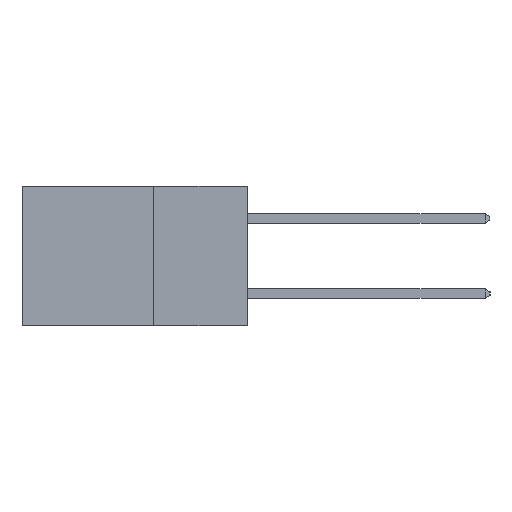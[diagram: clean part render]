
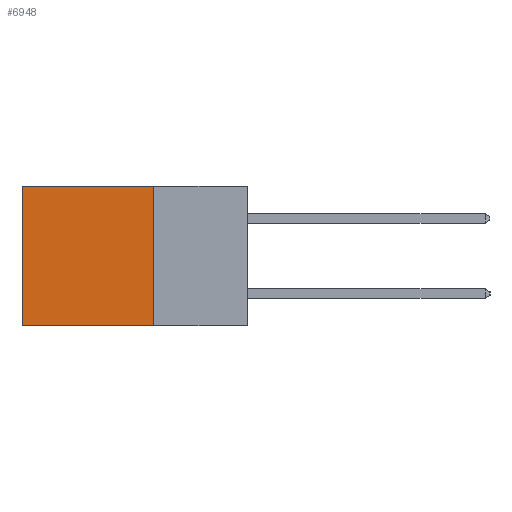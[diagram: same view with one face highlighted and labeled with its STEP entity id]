
A CAD part, left-side view. The second image highlights one B-rep face of the part: STEP entity #6948.
In plain terms, the highlighted planar face has unit normal (-1, 0, 0).
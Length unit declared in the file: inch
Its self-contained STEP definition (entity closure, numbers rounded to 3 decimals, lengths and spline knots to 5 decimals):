
#312 = CARTESIAN_POINT ( 'NONE',  ( 0.2615, 0.6, 0. ) ) ;
#363 = CARTESIAN_POINT ( 'NONE',  ( 0.2615, 0.6, -0.37 ) ) ;
#1145 = LINE ( 'NONE', #12063, #11334 ) ;
#1203 = EDGE_CURVE ( 'NONE', #11865, #4713, #4015, .T. ) ;
#1374 = VECTOR ( 'NONE', #1829, 39.37008 ) ;
#1567 = EDGE_LOOP ( 'NONE', ( #10245, #12551, #6251, #4119 ) ) ;
#1829 = DIRECTION ( 'NONE',  ( 0., 0., -1. ) ) ;
#2162 = CARTESIAN_POINT ( 'NONE',  ( 0.2615, 0.25, -0.37 ) ) ;
#2257 = VERTEX_POINT ( 'NONE', #3332 ) ;
#2989 = CARTESIAN_POINT ( 'NONE',  ( 0.2615, 0.25, -0.37 ) ) ;
#3332 = CARTESIAN_POINT ( 'NONE',  ( 0.2615, 0.25, 0. ) ) ;
#3408 = CARTESIAN_POINT ( 'NONE',  ( 0.2615, 0.6, -0.37 ) ) ;
#4015 = LINE ( 'NONE', #3408, #1374 ) ;
#4036 = DIRECTION ( 'NONE',  ( 1., 0., 0. ) ) ;
#4119 = ORIENTED_EDGE ( 'NONE', *, *, #5743, .T. ) ;
#4584 = VECTOR ( 'NONE', #8524, 39.37008 ) ;
#4713 = VERTEX_POINT ( 'NONE', #363 ) ;
#5154 = DIRECTION ( 'NONE',  ( 0., 1., 0. ) ) ;
#5445 = EDGE_CURVE ( 'NONE', #2257, #11313, #7203, .T. ) ;
#5727 = EDGE_CURVE ( 'NONE', #11313, #4713, #7041, .T. ) ;
#5743 = EDGE_CURVE ( 'NONE', #2257, #11865, #1145, .T. ) ;
#6251 = ORIENTED_EDGE ( 'NONE', *, *, #5445, .F. ) ;
#6948 = ADVANCED_FACE ( 'NONE', ( #12265 ), #8945, .F. ) ;
#7041 = LINE ( 'NONE', #2162, #9352 ) ;
#7203 = LINE ( 'NONE', #10454, #4584 ) ;
#8087 = DIRECTION ( 'NONE',  ( 0., 1., 0. ) ) ;
#8524 = DIRECTION ( 'NONE',  ( 0., 0., -1. ) ) ;
#8945 = PLANE ( 'NONE',  #11188 ) ;
#9352 = VECTOR ( 'NONE', #8087, 39.37008 ) ;
#10245 = ORIENTED_EDGE ( 'NONE', *, *, #1203, .T. ) ;
#10454 = CARTESIAN_POINT ( 'NONE',  ( 0.2615, 0.25, -0.37 ) ) ;
#10908 = DIRECTION ( 'NONE',  ( 0., 0., -1. ) ) ;
#11188 = AXIS2_PLACEMENT_3D ( 'NONE', #2989, #4036, #10908 ) ;
#11313 = VERTEX_POINT ( 'NONE', #12328 ) ;
#11334 = VECTOR ( 'NONE', #5154, 39.37008 ) ;
#11865 = VERTEX_POINT ( 'NONE', #312 ) ;
#12063 = CARTESIAN_POINT ( 'NONE',  ( 0.2615, 0.25, 0. ) ) ;
#12265 = FACE_OUTER_BOUND ( 'NONE', #1567, .T. ) ;
#12328 = CARTESIAN_POINT ( 'NONE',  ( 0.2615, 0.25, -0.37 ) ) ;
#12551 = ORIENTED_EDGE ( 'NONE', *, *, #5727, .F. ) ;
